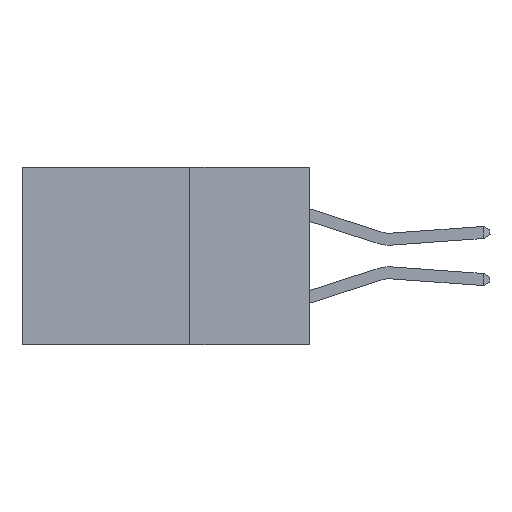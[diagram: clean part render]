
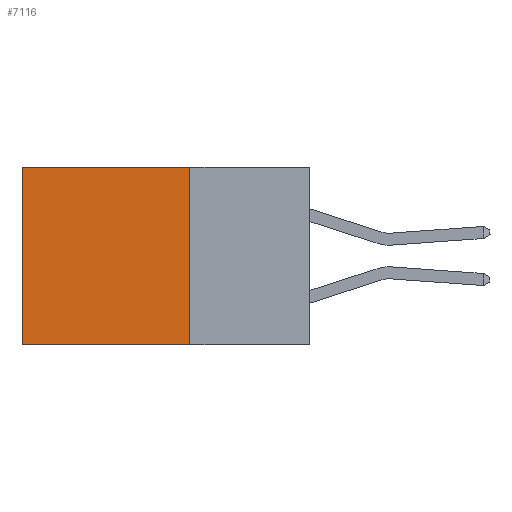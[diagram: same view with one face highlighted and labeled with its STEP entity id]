
A CAD part, left-side view. The second image highlights one B-rep face of the part: STEP entity #7116.
In plain terms, the highlighted planar face has unit normal (-1, 0, 0).
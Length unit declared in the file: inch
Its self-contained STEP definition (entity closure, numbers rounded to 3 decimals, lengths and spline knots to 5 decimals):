
#92 = VECTOR ( 'NONE', #8496, 39.37008 ) ;
#104 = VERTEX_POINT ( 'NONE', #2952 ) ;
#254 = EDGE_CURVE ( 'NONE', #11010, #104, #8052, .T. ) ;
#347 = CARTESIAN_POINT ( 'NONE',  ( 0.2615, 0.25, -0.37 ) ) ;
#613 = DIRECTION ( 'NONE',  ( 0., 1., 0. ) ) ;
#743 = CARTESIAN_POINT ( 'NONE',  ( 0.2615, 0.25, -0.37 ) ) ;
#1049 = EDGE_CURVE ( 'NONE', #4384, #12115, #10221, .T. ) ;
#2220 = DIRECTION ( 'NONE',  ( 0., 0., -1. ) ) ;
#2258 = CARTESIAN_POINT ( 'NONE',  ( 0.2615, 0.6, 0. ) ) ;
#2273 = PLANE ( 'NONE',  #2472 ) ;
#2327 = CARTESIAN_POINT ( 'NONE',  ( 0.2615, 0.25, -0.37 ) ) ;
#2345 = DIRECTION ( 'NONE',  ( 1., 0., 0. ) ) ;
#2472 = AXIS2_PLACEMENT_3D ( 'NONE', #2327, #2345, #2220 ) ;
#2952 = CARTESIAN_POINT ( 'NONE',  ( 0.2615, 0.6, -0.37 ) ) ;
#3234 = ORIENTED_EDGE ( 'NONE', *, *, #6715, .T. ) ;
#3433 = VECTOR ( 'NONE', #5950, 39.37008 ) ;
#4384 = VERTEX_POINT ( 'NONE', #8130 ) ;
#5950 = DIRECTION ( 'NONE',  ( 0., 1., 0. ) ) ;
#5956 = LINE ( 'NONE', #743, #8420 ) ;
#6019 = CARTESIAN_POINT ( 'NONE',  ( 0.2615, 0.25, 0. ) ) ;
#6113 = CARTESIAN_POINT ( 'NONE',  ( 0.2615, 0.25, -0.37 ) ) ;
#6715 = EDGE_CURVE ( 'NONE', #4384, #11010, #10762, .T. ) ;
#7116 = ADVANCED_FACE ( 'NONE', ( #9528 ), #2273, .F. ) ;
#7246 = EDGE_CURVE ( 'NONE', #12115, #104, #5956, .T. ) ;
#7313 = CARTESIAN_POINT ( 'NONE',  ( 0.2615, 0.6, -0.37 ) ) ;
#7356 = EDGE_LOOP ( 'NONE', ( #8766, #9988, #7479, #3234 ) ) ;
#7479 = ORIENTED_EDGE ( 'NONE', *, *, #1049, .F. ) ;
#8052 = LINE ( 'NONE', #7313, #92 ) ;
#8130 = CARTESIAN_POINT ( 'NONE',  ( 0.2615, 0.25, 0. ) ) ;
#8420 = VECTOR ( 'NONE', #613, 39.37008 ) ;
#8496 = DIRECTION ( 'NONE',  ( 0., 0., -1. ) ) ;
#8766 = ORIENTED_EDGE ( 'NONE', *, *, #254, .T. ) ;
#9528 = FACE_OUTER_BOUND ( 'NONE', #7356, .T. ) ;
#9988 = ORIENTED_EDGE ( 'NONE', *, *, #7246, .F. ) ;
#10106 = DIRECTION ( 'NONE',  ( 0., 0., -1. ) ) ;
#10221 = LINE ( 'NONE', #347, #12156 ) ;
#10762 = LINE ( 'NONE', #6019, #3433 ) ;
#11010 = VERTEX_POINT ( 'NONE', #2258 ) ;
#12115 = VERTEX_POINT ( 'NONE', #6113 ) ;
#12156 = VECTOR ( 'NONE', #10106, 39.37008 ) ;
